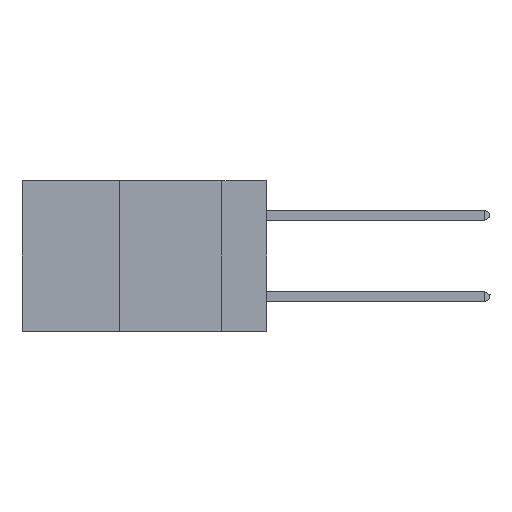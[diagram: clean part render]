
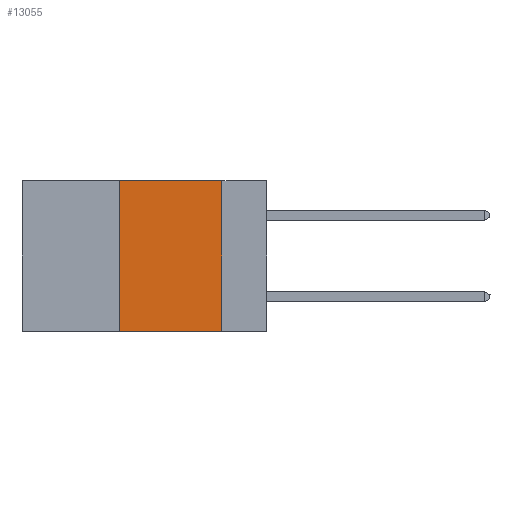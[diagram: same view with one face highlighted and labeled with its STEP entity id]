
A CAD part, left-side view. The second image highlights one B-rep face of the part: STEP entity #13055.
In plain terms, the highlighted planar face has unit normal (-1, 0, 0).
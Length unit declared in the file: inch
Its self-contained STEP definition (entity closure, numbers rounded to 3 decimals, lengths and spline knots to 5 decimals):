
#626 = ORIENTED_EDGE ( 'NONE', *, *, #7683, .F. ) ;
#854 = CARTESIAN_POINT ( 'NONE',  ( 0., 0.11, 0. ) ) ;
#1035 = FACE_OUTER_BOUND ( 'NONE', #10333, .T. ) ;
#1101 = DIRECTION ( 'NONE',  ( 1., 0., 0. ) ) ;
#1311 = CARTESIAN_POINT ( 'NONE',  ( 0., 0.36, -0.37 ) ) ;
#1607 = CARTESIAN_POINT ( 'NONE',  ( 0., 0.6, 0. ) ) ;
#1728 = VERTEX_POINT ( 'NONE', #13475 ) ;
#2220 = PLANE ( 'NONE',  #9785 ) ;
#3164 = DIRECTION ( 'NONE',  ( 0., 0., 1. ) ) ;
#5019 = VECTOR ( 'NONE', #3164, 39.37008 ) ;
#5562 = EDGE_CURVE ( 'NONE', #6515, #6084, #8317, .T. ) ;
#5633 = DIRECTION ( 'NONE',  ( 0., 0., -1. ) ) ;
#6084 = VERTEX_POINT ( 'NONE', #854 ) ;
#6515 = VERTEX_POINT ( 'NONE', #13109 ) ;
#6751 = CARTESIAN_POINT ( 'NONE',  ( 0., 0.6, 0. ) ) ;
#6947 = CARTESIAN_POINT ( 'NONE',  ( 0., 0.11, 0. ) ) ;
#7060 = ORIENTED_EDGE ( 'NONE', *, *, #5562, .F. ) ;
#7249 = DIRECTION ( 'NONE',  ( 0., 0., -1. ) ) ;
#7683 = EDGE_CURVE ( 'NONE', #6084, #1728, #11701, .T. ) ;
#7912 = DIRECTION ( 'NONE',  ( 0., -1., 0. ) ) ;
#8101 = VECTOR ( 'NONE', #7249, 39.37008 ) ;
#8239 = DIRECTION ( 'NONE',  ( 0., -1., 0. ) ) ;
#8317 = LINE ( 'NONE', #1607, #11595 ) ;
#8705 = LINE ( 'NONE', #13239, #14502 ) ;
#9785 = AXIS2_PLACEMENT_3D ( 'NONE', #6751, #1101, #5633 ) ;
#10111 = ORIENTED_EDGE ( 'NONE', *, *, #14169, .F. ) ;
#10172 = CARTESIAN_POINT ( 'NONE',  ( 0., 0.36, 0. ) ) ;
#10324 = LINE ( 'NONE', #10172, #5019 ) ;
#10333 = EDGE_LOOP ( 'NONE', ( #626, #7060, #10111, #12769 ) ) ;
#11595 = VECTOR ( 'NONE', #8239, 39.37008 ) ;
#11701 = LINE ( 'NONE', #6947, #8101 ) ;
#11999 = EDGE_CURVE ( 'NONE', #13526, #1728, #8705, .T. ) ;
#12769 = ORIENTED_EDGE ( 'NONE', *, *, #11999, .T. ) ;
#13055 = ADVANCED_FACE ( 'NONE', ( #1035 ), #2220, .F. ) ;
#13109 = CARTESIAN_POINT ( 'NONE',  ( 0., 0.36, 0. ) ) ;
#13239 = CARTESIAN_POINT ( 'NONE',  ( 0., 0.6, -0.37 ) ) ;
#13475 = CARTESIAN_POINT ( 'NONE',  ( 0., 0.11, -0.37 ) ) ;
#13526 = VERTEX_POINT ( 'NONE', #1311 ) ;
#14169 = EDGE_CURVE ( 'NONE', #13526, #6515, #10324, .T. ) ;
#14502 = VECTOR ( 'NONE', #7912, 39.37008 ) ;
